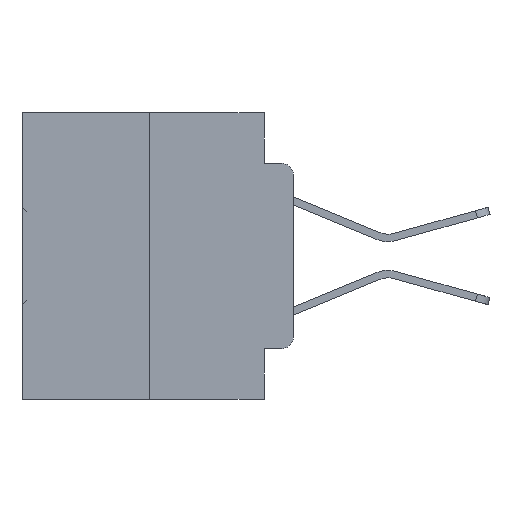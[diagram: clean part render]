
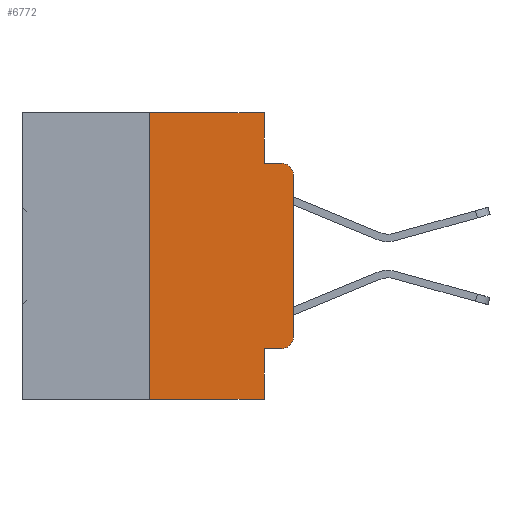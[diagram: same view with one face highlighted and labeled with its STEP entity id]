
A CAD part, left-side view. The second image highlights one B-rep face of the part: STEP entity #6772.
In plain terms, the highlighted planar face has unit normal (-1, 0, 0).
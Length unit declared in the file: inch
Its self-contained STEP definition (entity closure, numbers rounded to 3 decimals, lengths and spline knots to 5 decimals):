
#465 = ORIENTED_EDGE ( 'NONE', *, *, #23543, .F. ) ;
#1350 = DIRECTION ( 'NONE',  ( 0., 0., -1. ) ) ;
#1419 = DIRECTION ( 'NONE',  ( -1., 0., 0. ) ) ;
#1586 = CARTESIAN_POINT ( 'NONE',  ( 0., 0.473, 0. ) ) ;
#2410 = LINE ( 'NONE', #7744, #16726 ) ;
#2835 = ORIENTED_EDGE ( 'NONE', *, *, #13969, .T. ) ;
#3245 = ORIENTED_EDGE ( 'NONE', *, *, #5126, .T. ) ;
#3425 = FACE_OUTER_BOUND ( 'NONE', #7264, .T. ) ;
#3478 = CARTESIAN_POINT ( 'NONE',  ( 0., 0.25, -0.5 ) ) ;
#3851 = AXIS2_PLACEMENT_3D ( 'NONE', #27179, #10641, #9327 ) ;
#3924 = CARTESIAN_POINT ( 'NONE',  ( 0., 0.02, -0.4115 ) ) ;
#4003 = ORIENTED_EDGE ( 'NONE', *, *, #8735, .T. ) ;
#4330 = DIRECTION ( 'NONE',  ( 0., -1., 0. ) ) ;
#4454 = ORIENTED_EDGE ( 'NONE', *, *, #25379, .F. ) ;
#4524 = VECTOR ( 'NONE', #4967, 39.37008 ) ;
#4614 = ORIENTED_EDGE ( 'NONE', *, *, #31458, .F. ) ;
#4717 = EDGE_CURVE ( 'NONE', #12404, #7147, #23600, .T. ) ;
#4755 = VERTEX_POINT ( 'NONE', #3924 ) ;
#4967 = DIRECTION ( 'NONE',  ( 0., 0., -1. ) ) ;
#5126 = EDGE_CURVE ( 'NONE', #33043, #4755, #19870, .T. ) ;
#5253 = CARTESIAN_POINT ( 'NONE',  ( 0., 0.051, -0.0885 ) ) ;
#5648 = VECTOR ( 'NONE', #25456, 39.37008 ) ;
#5887 = LINE ( 'NONE', #23171, #22987 ) ;
#5921 = CARTESIAN_POINT ( 'NONE',  ( 0., 0.25, 0. ) ) ;
#6112 = ORIENTED_EDGE ( 'NONE', *, *, #4717, .T. ) ;
#6735 = EDGE_CURVE ( 'NONE', #4755, #31853, #25546, .T. ) ;
#6772 = ADVANCED_FACE ( 'NONE', ( #3425 ), #29503, .F. ) ;
#7147 = VERTEX_POINT ( 'NONE', #28821 ) ;
#7264 = EDGE_LOOP ( 'NONE', ( #4003, #6112, #4614, #32091, #4454, #465, #2835, #27368, #3245, #11396 ) ) ;
#7271 = LINE ( 'NONE', #8885, #21409 ) ;
#7744 = CARTESIAN_POINT ( 'NONE',  ( 0., 0.051, 0. ) ) ;
#7960 = DIRECTION ( 'NONE',  ( 0., -1., 0. ) ) ;
#8080 = AXIS2_PLACEMENT_3D ( 'NONE', #22709, #1419, #1350 ) ;
#8378 = DIRECTION ( 'NONE',  ( 0., 0., 1. ) ) ;
#8735 = EDGE_CURVE ( 'NONE', #31853, #12404, #7271, .T. ) ;
#8885 = CARTESIAN_POINT ( 'NONE',  ( 0., 0., 0. ) ) ;
#9327 = DIRECTION ( 'NONE',  ( 0., 0., -1. ) ) ;
#9559 = CARTESIAN_POINT ( 'NONE',  ( 0., 0.051, -0.4115 ) ) ;
#10070 = VERTEX_POINT ( 'NONE', #21941 ) ;
#10641 = DIRECTION ( 'NONE',  ( 1., 0., 0. ) ) ;
#11347 = CARTESIAN_POINT ( 'NONE',  ( 0., 0.051, -0.0885 ) ) ;
#11396 = ORIENTED_EDGE ( 'NONE', *, *, #6735, .T. ) ;
#12284 = EDGE_CURVE ( 'NONE', #25597, #31639, #30280, .T. ) ;
#12404 = VERTEX_POINT ( 'NONE', #16340 ) ;
#13969 = EDGE_CURVE ( 'NONE', #33457, #10070, #5887, .T. ) ;
#15298 = VECTOR ( 'NONE', #4330, 39.37008 ) ;
#15612 = DIRECTION ( 'NONE',  ( 0., 0., 1. ) ) ;
#16340 = CARTESIAN_POINT ( 'NONE',  ( 0., 0., -0.1085 ) ) ;
#16726 = VECTOR ( 'NONE', #21015, 39.37008 ) ;
#17106 = VECTOR ( 'NONE', #15612, 39.37008 ) ;
#18060 = CARTESIAN_POINT ( 'NONE',  ( 0., 0.25, 0. ) ) ;
#19870 = LINE ( 'NONE', #9559, #5648 ) ;
#20036 = CARTESIAN_POINT ( 'NONE',  ( 0., 0.02, -0.3915 ) ) ;
#21015 = DIRECTION ( 'NONE',  ( 0., 0., -1. ) ) ;
#21409 = VECTOR ( 'NONE', #8378, 39.37008 ) ;
#21941 = CARTESIAN_POINT ( 'NONE',  ( 0., 0.051, -0.5 ) ) ;
#22709 = CARTESIAN_POINT ( 'NONE',  ( 0., 0.02, -0.1085 ) ) ;
#22987 = VECTOR ( 'NONE', #25831, 39.37008 ) ;
#23040 = LINE ( 'NONE', #5253, #29214 ) ;
#23171 = CARTESIAN_POINT ( 'NONE',  ( 0., 0.473, -0.5 ) ) ;
#23543 = EDGE_CURVE ( 'NONE', #33457, #26642, #31085, .T. ) ;
#23600 = CIRCLE ( 'NONE', #8080, 0.02 ) ;
#25379 = EDGE_CURVE ( 'NONE', #26642, #25597, #29311, .T. ) ;
#25456 = DIRECTION ( 'NONE',  ( 0., -1., 0. ) ) ;
#25546 = CIRCLE ( 'NONE', #29452, 0.02 ) ;
#25597 = VERTEX_POINT ( 'NONE', #29633 ) ;
#25831 = DIRECTION ( 'NONE',  ( 0., -1., 0. ) ) ;
#26259 = CARTESIAN_POINT ( 'NONE',  ( 0., 0.051, 0. ) ) ;
#26642 = VERTEX_POINT ( 'NONE', #5921 ) ;
#27179 = CARTESIAN_POINT ( 'NONE',  ( 0., 0.473, 0. ) ) ;
#27368 = ORIENTED_EDGE ( 'NONE', *, *, #27729, .F. ) ;
#27729 = EDGE_CURVE ( 'NONE', #33043, #10070, #2410, .T. ) ;
#28212 = DIRECTION ( 'NONE',  ( 0., 0., -1. ) ) ;
#28821 = CARTESIAN_POINT ( 'NONE',  ( 0., 0.02, -0.0885 ) ) ;
#29214 = VECTOR ( 'NONE', #7960, 39.37008 ) ;
#29311 = LINE ( 'NONE', #1586, #15298 ) ;
#29452 = AXIS2_PLACEMENT_3D ( 'NONE', #20036, #34045, #28212 ) ;
#29503 = PLANE ( 'NONE',  #3851 ) ;
#29633 = CARTESIAN_POINT ( 'NONE',  ( 0., 0.051, 0. ) ) ;
#30280 = LINE ( 'NONE', #26259, #4524 ) ;
#30763 = CARTESIAN_POINT ( 'NONE',  ( 0., 0., -0.3915 ) ) ;
#31039 = CARTESIAN_POINT ( 'NONE',  ( 0., 0.051, -0.4115 ) ) ;
#31085 = LINE ( 'NONE', #18060, #17106 ) ;
#31458 = EDGE_CURVE ( 'NONE', #31639, #7147, #23040, .T. ) ;
#31639 = VERTEX_POINT ( 'NONE', #11347 ) ;
#31853 = VERTEX_POINT ( 'NONE', #30763 ) ;
#32091 = ORIENTED_EDGE ( 'NONE', *, *, #12284, .F. ) ;
#33043 = VERTEX_POINT ( 'NONE', #31039 ) ;
#33457 = VERTEX_POINT ( 'NONE', #3478 ) ;
#34045 = DIRECTION ( 'NONE',  ( -1., 0., 0. ) ) ;
